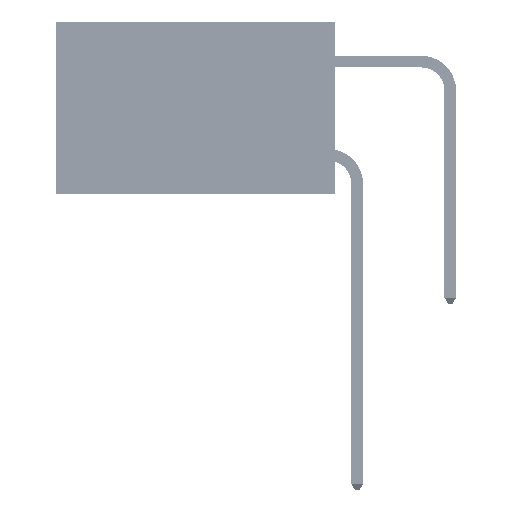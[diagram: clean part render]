
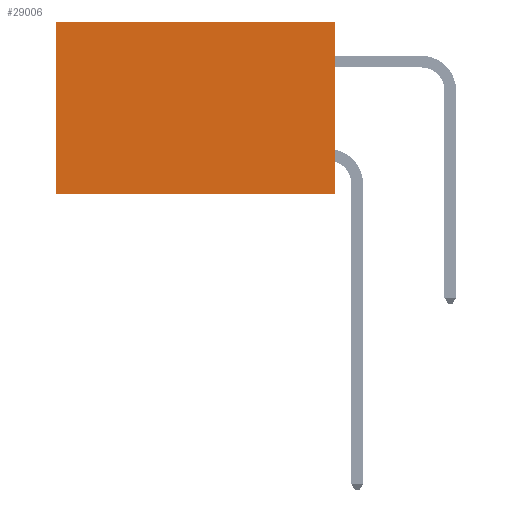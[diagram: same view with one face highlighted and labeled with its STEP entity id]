
A CAD part, left-side view. The second image highlights one B-rep face of the part: STEP entity #29006.
In plain terms, the highlighted planar face has unit normal (-1, 0, 0).
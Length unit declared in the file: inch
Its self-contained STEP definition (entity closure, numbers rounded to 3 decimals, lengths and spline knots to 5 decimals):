
#497 = DIRECTION ( 'NONE',  ( 0., 0., -1. ) ) ;
#1611 = ORIENTED_EDGE ( 'NONE', *, *, #12873, .T. ) ;
#2671 = VERTEX_POINT ( 'NONE', #38880 ) ;
#2817 = CARTESIAN_POINT ( 'NONE',  ( 0.2875, 0., -0.37 ) ) ;
#4739 = VECTOR ( 'NONE', #17950, 39.37008 ) ;
#5752 = DIRECTION ( 'NONE',  ( 0., 0., -1. ) ) ;
#7179 = EDGE_CURVE ( 'NONE', #19614, #2671, #42407, .T. ) ;
#7639 = DIRECTION ( 'NONE',  ( 0., 1., 0. ) ) ;
#11626 = VERTEX_POINT ( 'NONE', #36436 ) ;
#12873 = EDGE_CURVE ( 'NONE', #11626, #19614, #31198, .T. ) ;
#14111 = FACE_OUTER_BOUND ( 'NONE', #28803, .T. ) ;
#15354 = LINE ( 'NONE', #37674, #4739 ) ;
#17289 = VECTOR ( 'NONE', #7639, 39.37008 ) ;
#17861 = ORIENTED_EDGE ( 'NONE', *, *, #7179, .T. ) ;
#17950 = DIRECTION ( 'NONE',  ( 0., 0., -1. ) ) ;
#17998 = ORIENTED_EDGE ( 'NONE', *, *, #45773, .F. ) ;
#19556 = CARTESIAN_POINT ( 'NONE',  ( 0.2875, 0., 0. ) ) ;
#19614 = VERTEX_POINT ( 'NONE', #38975 ) ;
#20283 = VERTEX_POINT ( 'NONE', #2817 ) ;
#21730 = CARTESIAN_POINT ( 'NONE',  ( 0.2875, 0.6, 0. ) ) ;
#22407 = ORIENTED_EDGE ( 'NONE', *, *, #26046, .F. ) ;
#23558 = DIRECTION ( 'NONE',  ( 0., 1., 0. ) ) ;
#24398 = DIRECTION ( 'NONE',  ( 1., 0., 0. ) ) ;
#26046 = EDGE_CURVE ( 'NONE', #20283, #2671, #38357, .T. ) ;
#27473 = CARTESIAN_POINT ( 'NONE',  ( 0.2875, 0., -0.37 ) ) ;
#28803 = EDGE_LOOP ( 'NONE', ( #17861, #22407, #17998, #1611 ) ) ;
#29006 = ADVANCED_FACE ( 'NONE', ( #14111 ), #36160, .F. ) ;
#29485 = VECTOR ( 'NONE', #5752, 39.37008 ) ;
#31198 = LINE ( 'NONE', #19556, #50819 ) ;
#36160 = PLANE ( 'NONE',  #45432 ) ;
#36436 = CARTESIAN_POINT ( 'NONE',  ( 0.2875, 0., 0. ) ) ;
#37674 = CARTESIAN_POINT ( 'NONE',  ( 0.2875, 0., 0. ) ) ;
#38357 = LINE ( 'NONE', #27473, #17289 ) ;
#38880 = CARTESIAN_POINT ( 'NONE',  ( 0.2875, 0.6, -0.37 ) ) ;
#38975 = CARTESIAN_POINT ( 'NONE',  ( 0.2875, 0.6, 0. ) ) ;
#42407 = LINE ( 'NONE', #21730, #29485 ) ;
#45432 = AXIS2_PLACEMENT_3D ( 'NONE', #47988, #24398, #497 ) ;
#45773 = EDGE_CURVE ( 'NONE', #11626, #20283, #15354, .T. ) ;
#47988 = CARTESIAN_POINT ( 'NONE',  ( 0.2875, 0., 0. ) ) ;
#50819 = VECTOR ( 'NONE', #23558, 39.37008 ) ;
